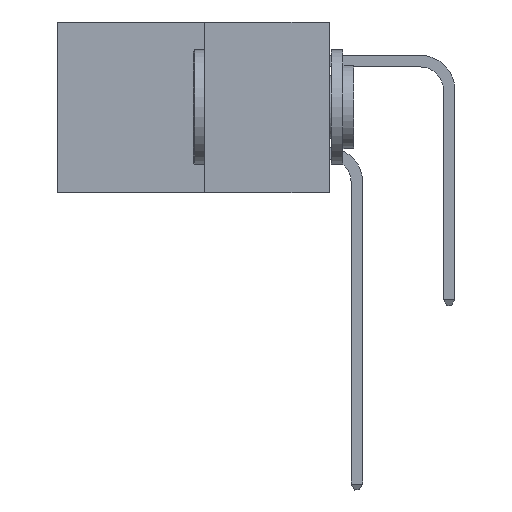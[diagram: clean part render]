
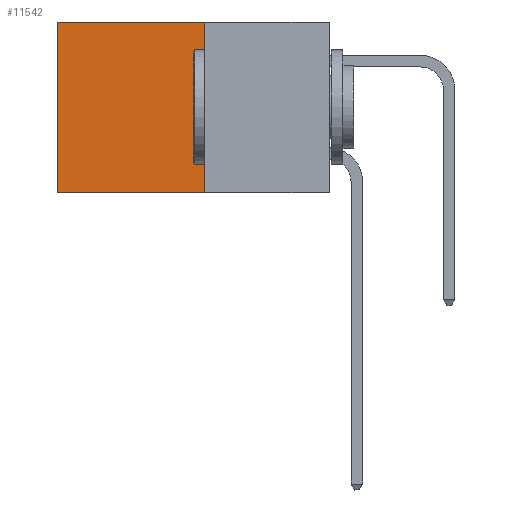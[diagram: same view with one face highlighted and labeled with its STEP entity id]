
A CAD part, left-side view. The second image highlights one B-rep face of the part: STEP entity #11542.
In plain terms, the highlighted planar face has unit normal (-1, 0, 0).
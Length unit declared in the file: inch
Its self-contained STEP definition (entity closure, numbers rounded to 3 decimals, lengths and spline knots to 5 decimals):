
#2315 = CARTESIAN_POINT ( 'NONE',  ( 0.277, 0.27, 0. ) ) ;
#2630 = ORIENTED_EDGE ( 'NONE', *, *, #12930, .F. ) ;
#3526 = AXIS2_PLACEMENT_3D ( 'NONE', #21965, #10544, #23864 ) ;
#3639 = VECTOR ( 'NONE', #13057, 39.37008 ) ;
#4586 = VERTEX_POINT ( 'NONE', #24284 ) ;
#4788 = PLANE ( 'NONE',  #3526 ) ;
#5363 = VECTOR ( 'NONE', #24031, 39.37008 ) ;
#5702 = VECTOR ( 'NONE', #6371, 39.37008 ) ;
#5759 = CARTESIAN_POINT ( 'NONE',  ( 0.277, 0.27, -0.37 ) ) ;
#6156 = EDGE_CURVE ( 'NONE', #22830, #11137, #19702, .T. ) ;
#6371 = DIRECTION ( 'NONE',  ( 0., 0., -1. ) ) ;
#6711 = ORIENTED_EDGE ( 'NONE', *, *, #7982, .T. ) ;
#7043 = CARTESIAN_POINT ( 'NONE',  ( 0.277, 0.27, 0. ) ) ;
#7280 = LINE ( 'NONE', #7043, #20103 ) ;
#7982 = EDGE_CURVE ( 'NONE', #4586, #13779, #21151, .T. ) ;
#9604 = LINE ( 'NONE', #20659, #3639 ) ;
#10544 = DIRECTION ( 'NONE',  ( 1., 0., 0. ) ) ;
#11073 = EDGE_CURVE ( 'NONE', #22830, #4586, #7280, .T. ) ;
#11137 = VERTEX_POINT ( 'NONE', #24379 ) ;
#11542 = ADVANCED_FACE ( 'NONE', ( #19477 ), #4788, .F. ) ;
#12179 = ORIENTED_EDGE ( 'NONE', *, *, #6156, .F. ) ;
#12930 = EDGE_CURVE ( 'NONE', #11137, #13779, #9604, .T. ) ;
#13057 = DIRECTION ( 'NONE',  ( 0., 1., 0. ) ) ;
#13779 = VERTEX_POINT ( 'NONE', #23300 ) ;
#18938 = EDGE_LOOP ( 'NONE', ( #6711, #2630, #12179, #20280 ) ) ;
#19477 = FACE_OUTER_BOUND ( 'NONE', #18938, .T. ) ;
#19702 = LINE ( 'NONE', #5759, #5702 ) ;
#20103 = VECTOR ( 'NONE', #24225, 39.37008 ) ;
#20280 = ORIENTED_EDGE ( 'NONE', *, *, #11073, .T. ) ;
#20659 = CARTESIAN_POINT ( 'NONE',  ( 0.277, 0.27, -0.37 ) ) ;
#21151 = LINE ( 'NONE', #24178, #5363 ) ;
#21965 = CARTESIAN_POINT ( 'NONE',  ( 0.277, 0.27, -0.37 ) ) ;
#22830 = VERTEX_POINT ( 'NONE', #2315 ) ;
#23300 = CARTESIAN_POINT ( 'NONE',  ( 0.277, 0.59, -0.37 ) ) ;
#23864 = DIRECTION ( 'NONE',  ( 0., 0., -1. ) ) ;
#24031 = DIRECTION ( 'NONE',  ( 0., 0., -1. ) ) ;
#24178 = CARTESIAN_POINT ( 'NONE',  ( 0.277, 0.59, -0.37 ) ) ;
#24225 = DIRECTION ( 'NONE',  ( 0., 1., 0. ) ) ;
#24284 = CARTESIAN_POINT ( 'NONE',  ( 0.277, 0.59, 0. ) ) ;
#24379 = CARTESIAN_POINT ( 'NONE',  ( 0.277, 0.27, -0.37 ) ) ;
